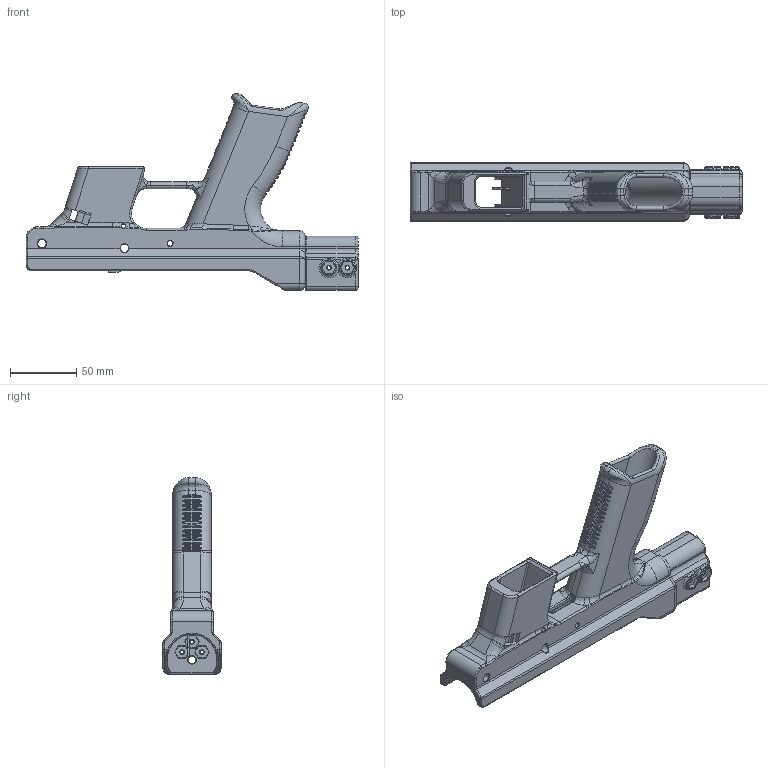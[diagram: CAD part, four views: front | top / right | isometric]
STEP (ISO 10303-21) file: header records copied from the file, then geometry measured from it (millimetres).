
FILE_DESCRIPTION(/* description */ (''),/* implementation_level */ '2;1');
FILE_NAME(/* name */ '2db2668f-834a-4ed3-80de-1a24cb0b059f.stp',/* time_stamp */ '2019-04-26T13:10:35-04:00',/* author */ ('suzuki450ltr'),/* organization */ (''),/* preprocessor_version */ 'ST-DEVELOPER v18',/* originating_system */ 'Autodesk Translation Framework v8.2.0.1029',/* authorisation */ '');
FILE_SCHEMA (('AUTOMOTIVE_DESIGN { 1 0 10303 214 3 1 1 }'));
Products named in the file (3): AB-10 Brace Reciever 3; Moddified Ejector; Brace Adapter
Assembly tree (2 placements, depth 2):
  AB-10 Brace Reciever 3
    Moddified Ejector
    Brace Adapter
Bounding box: 250.98 x 44 x 148.84 mm (x, y, z)
Volume: 254702.5 mm3; surface area: 92807.4 mm2
Topology: 3 solids, 3 shells, 1168 faces, 2845 edges, 1646 vertices
Faces by surface type: bspline 412, cylinder 322, plane 285, torus 101, cone 42, sphere 6
Full cylindrical faces by diameter (mm): 3 x10, 3.175 x3, 4 x2, 5.5 x1, 6.3 x5, 6.5 x1, 10 x5, 12 x4, 26 x1
Entity records: 48240 total; most frequent: CARTESIAN_POINT 22510, ORIENTED_EDGE 5644, DIRECTION 4970, EDGE_CURVE 2822, AXIS2_PLACEMENT_3D 1980, VERTEX_POINT 1651, EDGE_LOOP 1213, FACE_OUTER_BOUND 1168
